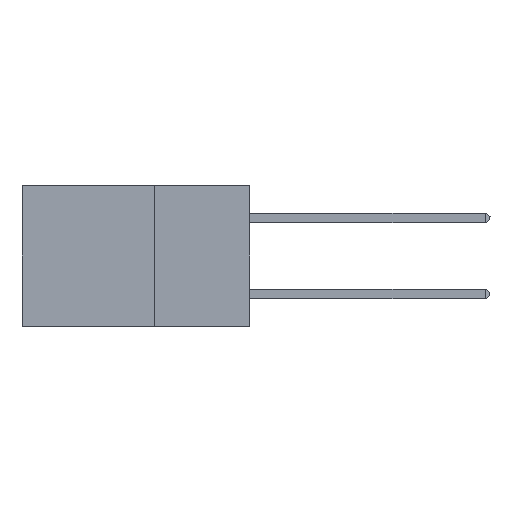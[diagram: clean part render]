
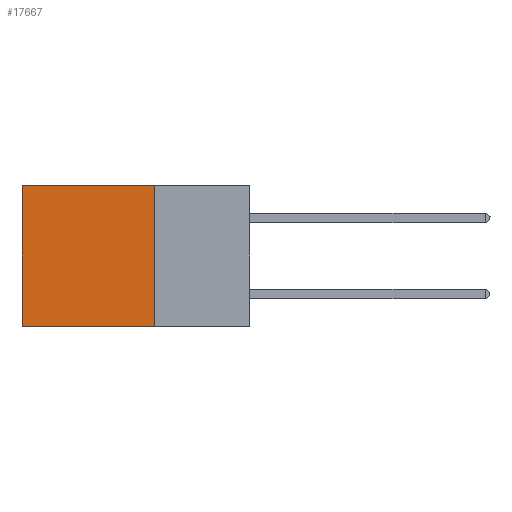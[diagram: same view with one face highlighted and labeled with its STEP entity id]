
A CAD part, left-side view. The second image highlights one B-rep face of the part: STEP entity #17667.
In plain terms, the highlighted planar face has unit normal (-1, 0, 0).
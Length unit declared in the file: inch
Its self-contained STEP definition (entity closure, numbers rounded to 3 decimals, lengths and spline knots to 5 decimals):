
#1026 = EDGE_CURVE ( 'NONE', #1351, #17945, #14490, .T. ) ;
#1062 = LINE ( 'NONE', #14813, #8046 ) ;
#1351 = VERTEX_POINT ( 'NONE', #11345 ) ;
#1680 = CARTESIAN_POINT ( 'NONE',  ( 0.2875, 0.6, -0.37 ) ) ;
#1966 = DIRECTION ( 'NONE',  ( 0., 0., -1. ) ) ;
#2507 = EDGE_CURVE ( 'NONE', #2622, #1351, #7726, .T. ) ;
#2622 = VERTEX_POINT ( 'NONE', #10002 ) ;
#3749 = DIRECTION ( 'NONE',  ( 1., 0., 0. ) ) ;
#4508 = ORIENTED_EDGE ( 'NONE', *, *, #13926, .T. ) ;
#4927 = CARTESIAN_POINT ( 'NONE',  ( 0.2875, 0.25, -0.37 ) ) ;
#5079 = DIRECTION ( 'NONE',  ( 0., 0., -1. ) ) ;
#5319 = PLANE ( 'NONE',  #11673 ) ;
#5581 = ORIENTED_EDGE ( 'NONE', *, *, #2507, .F. ) ;
#6130 = FACE_OUTER_BOUND ( 'NONE', #8183, .T. ) ;
#6328 = ORIENTED_EDGE ( 'NONE', *, *, #1026, .F. ) ;
#7726 = LINE ( 'NONE', #11241, #11824 ) ;
#8046 = VECTOR ( 'NONE', #10780, 39.37008 ) ;
#8183 = EDGE_LOOP ( 'NONE', ( #10012, #6328, #5581, #4508 ) ) ;
#9105 = LINE ( 'NONE', #15798, #11041 ) ;
#10002 = CARTESIAN_POINT ( 'NONE',  ( 0.2875, 0.25, 0. ) ) ;
#10012 = ORIENTED_EDGE ( 'NONE', *, *, #14342, .T. ) ;
#10041 = CARTESIAN_POINT ( 'NONE',  ( 0.2875, 0.6, 0. ) ) ;
#10780 = DIRECTION ( 'NONE',  ( 0., 1., 0. ) ) ;
#11041 = VECTOR ( 'NONE', #1966, 39.37008 ) ;
#11241 = CARTESIAN_POINT ( 'NONE',  ( 0.2875, 0.25, 0. ) ) ;
#11345 = CARTESIAN_POINT ( 'NONE',  ( 0.2875, 0.25, -0.37 ) ) ;
#11673 = AXIS2_PLACEMENT_3D ( 'NONE', #12113, #3749, #5079 ) ;
#11824 = VECTOR ( 'NONE', #12525, 39.37008 ) ;
#12113 = CARTESIAN_POINT ( 'NONE',  ( 0.2875, 0.25, 0. ) ) ;
#12525 = DIRECTION ( 'NONE',  ( 0., 0., -1. ) ) ;
#13279 = VERTEX_POINT ( 'NONE', #10041 ) ;
#13926 = EDGE_CURVE ( 'NONE', #2622, #13279, #1062, .T. ) ;
#14342 = EDGE_CURVE ( 'NONE', #13279, #17945, #9105, .T. ) ;
#14490 = LINE ( 'NONE', #4927, #16867 ) ;
#14813 = CARTESIAN_POINT ( 'NONE',  ( 0.2875, 0.25, 0. ) ) ;
#15798 = CARTESIAN_POINT ( 'NONE',  ( 0.2875, 0.6, 0. ) ) ;
#16867 = VECTOR ( 'NONE', #17491, 39.37008 ) ;
#17491 = DIRECTION ( 'NONE',  ( 0., 1., 0. ) ) ;
#17667 = ADVANCED_FACE ( 'NONE', ( #6130 ), #5319, .F. ) ;
#17945 = VERTEX_POINT ( 'NONE', #1680 ) ;
